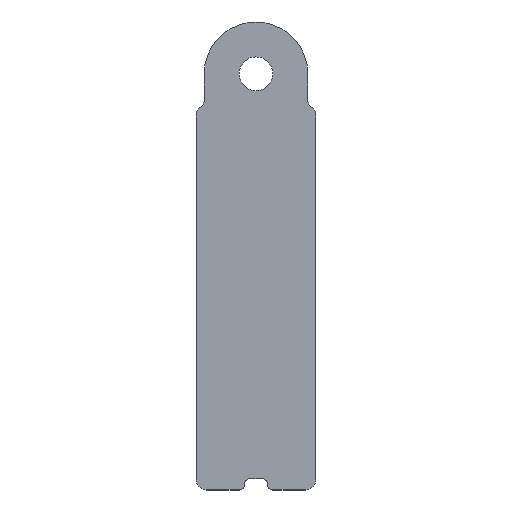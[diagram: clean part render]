
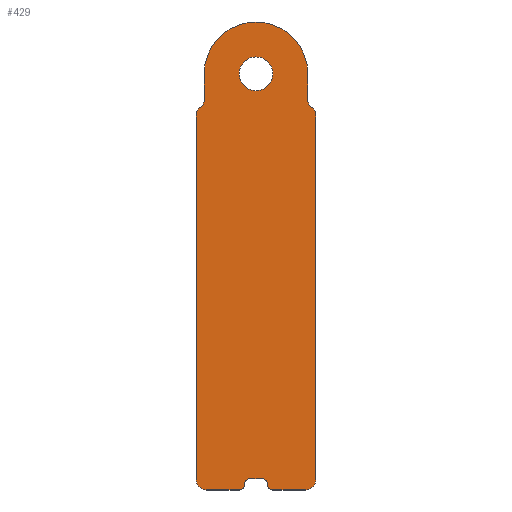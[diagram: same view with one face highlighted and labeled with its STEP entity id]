
A CAD part, top view. The second image highlights one B-rep face of the part: STEP entity #429.
In plain terms, the highlighted planar face has unit normal (0, 0, 1).
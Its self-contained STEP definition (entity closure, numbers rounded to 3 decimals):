
#16=FACE_BOUND('',#61,.T.);
#21=PLANE('',#482);
#36=FACE_OUTER_BOUND('',#60,.T.);
#60=EDGE_LOOP('',(#332,#333,#334,#335,#336,#337,#338,#339,#340,#341,#342,
#343,#344,#345,#346,#347,#348,#349,#350,#351));
#61=EDGE_LOOP('',(#352));
#87=LINE('',#692,#126);
#92=LINE('',#705,#131);
#95=LINE('',#714,#134);
#97=LINE('',#718,#136);
#98=LINE('',#722,#137);
#99=LINE('',#728,#138);
#100=LINE('',#732,#139);
#101=LINE('',#738,#140);
#102=LINE('',#740,#141);
#126=VECTOR('',#550,10.);
#131=VECTOR('',#565,10.);
#134=VECTOR('',#574,10.);
#136=VECTOR('',#578,10.);
#137=VECTOR('',#581,10.);
#138=VECTOR('',#586,10.);
#139=VECTOR('',#589,10.);
#140=VECTOR('',#594,10.);
#141=VECTOR('',#597,10.);
#154=CIRCLE('',#459,0.5);
#167=CIRCLE('',#475,0.5);
#168=CIRCLE('',#477,0.5);
#169=CIRCLE('',#480,0.5);
#170=CIRCLE('',#483,1.);
#171=CIRCLE('',#484,0.75);
#172=CIRCLE('',#485,0.75);
#173=CIRCLE('',#486,4.9);
#174=CIRCLE('',#487,0.75);
#175=CIRCLE('',#488,0.75);
#176=CIRCLE('',#489,1.);
#177=CIRCLE('',#490,1.6);
#178=VERTEX_POINT('',#642);
#179=VERTEX_POINT('',#643);
#201=VERTEX_POINT('',#691);
#202=VERTEX_POINT('',#695);
#203=VERTEX_POINT('',#699);
#204=VERTEX_POINT('',#701);
#205=VERTEX_POINT('',#707);
#206=VERTEX_POINT('',#708);
#207=VERTEX_POINT('',#713);
#208=VERTEX_POINT('',#717);
#209=VERTEX_POINT('',#719);
#210=VERTEX_POINT('',#721);
#211=VERTEX_POINT('',#723);
#212=VERTEX_POINT('',#725);
#213=VERTEX_POINT('',#727);
#214=VERTEX_POINT('',#729);
#215=VERTEX_POINT('',#731);
#216=VERTEX_POINT('',#733);
#217=VERTEX_POINT('',#735);
#218=VERTEX_POINT('',#737);
#219=VERTEX_POINT('',#741);
#220=EDGE_CURVE('',#178,#179,#154,.T.);
#244=EDGE_CURVE('',#201,#179,#87,.T.);
#246=EDGE_CURVE('',#201,#202,#167,.T.);
#249=EDGE_CURVE('',#203,#204,#168,.T.);
#251=EDGE_CURVE('',#203,#202,#92,.T.);
#252=EDGE_CURVE('',#205,#206,#169,.T.);
#255=EDGE_CURVE('',#207,#206,#95,.T.);
#257=EDGE_CURVE('',#178,#208,#97,.T.);
#258=EDGE_CURVE('',#209,#208,#170,.T.);
#259=EDGE_CURVE('',#209,#210,#98,.T.);
#260=EDGE_CURVE('',#211,#210,#171,.T.);
#261=EDGE_CURVE('',#212,#211,#172,.T.);
#262=EDGE_CURVE('',#212,#213,#99,.T.);
#263=EDGE_CURVE('',#213,#214,#173,.T.);
#264=EDGE_CURVE('',#214,#215,#100,.T.);
#265=EDGE_CURVE('',#216,#215,#174,.T.);
#266=EDGE_CURVE('',#217,#216,#175,.T.);
#267=EDGE_CURVE('',#217,#218,#101,.T.);
#268=EDGE_CURVE('',#207,#218,#176,.T.);
#269=EDGE_CURVE('',#205,#204,#102,.T.);
#270=EDGE_CURVE('',#219,#219,#177,.T.);
#332=ORIENTED_EDGE('',*,*,#220,.F.);
#333=ORIENTED_EDGE('',*,*,#257,.T.);
#334=ORIENTED_EDGE('',*,*,#258,.F.);
#335=ORIENTED_EDGE('',*,*,#259,.T.);
#336=ORIENTED_EDGE('',*,*,#260,.F.);
#337=ORIENTED_EDGE('',*,*,#261,.F.);
#338=ORIENTED_EDGE('',*,*,#262,.T.);
#339=ORIENTED_EDGE('',*,*,#263,.T.);
#340=ORIENTED_EDGE('',*,*,#264,.T.);
#341=ORIENTED_EDGE('',*,*,#265,.F.);
#342=ORIENTED_EDGE('',*,*,#266,.F.);
#343=ORIENTED_EDGE('',*,*,#267,.T.);
#344=ORIENTED_EDGE('',*,*,#268,.F.);
#345=ORIENTED_EDGE('',*,*,#255,.T.);
#346=ORIENTED_EDGE('',*,*,#252,.F.);
#347=ORIENTED_EDGE('',*,*,#269,.T.);
#348=ORIENTED_EDGE('',*,*,#249,.F.);
#349=ORIENTED_EDGE('',*,*,#251,.T.);
#350=ORIENTED_EDGE('',*,*,#246,.F.);
#351=ORIENTED_EDGE('',*,*,#244,.T.);
#352=ORIENTED_EDGE('',*,*,#270,.T.);
#429=ADVANCED_FACE('',(#36,#16),#21,.T.);
#459=AXIS2_PLACEMENT_3D('',#644,#509,#510);
#475=AXIS2_PLACEMENT_3D('',#696,#554,#555);
#477=AXIS2_PLACEMENT_3D('',#702,#560,#561);
#480=AXIS2_PLACEMENT_3D('',#709,#568,#569);
#482=AXIS2_PLACEMENT_3D('',#716,#576,#577);
#483=AXIS2_PLACEMENT_3D('',#720,#579,#580);
#484=AXIS2_PLACEMENT_3D('',#724,#582,#583);
#485=AXIS2_PLACEMENT_3D('',#726,#584,#585);
#486=AXIS2_PLACEMENT_3D('',#730,#587,#588);
#487=AXIS2_PLACEMENT_3D('',#734,#590,#591);
#488=AXIS2_PLACEMENT_3D('',#736,#592,#593);
#489=AXIS2_PLACEMENT_3D('',#739,#595,#596);
#490=AXIS2_PLACEMENT_3D('',#742,#598,#599);
#509=DIRECTION('center_axis',(0.,0.,-1.));
#510=DIRECTION('ref_axis',(-0.707,-0.707,0.));
#550=DIRECTION('',(0.,-1.,0.));
#554=DIRECTION('center_axis',(0.,0.,1.));
#555=DIRECTION('ref_axis',(0.707,0.707,0.));
#560=DIRECTION('center_axis',(0.,0.,1.));
#561=DIRECTION('ref_axis',(-0.707,0.707,0.));
#565=DIRECTION('',(1.,0.,0.));
#568=DIRECTION('center_axis',(0.,0.,-1.));
#569=DIRECTION('ref_axis',(0.707,-0.707,0.));
#574=DIRECTION('',(1.,0.,0.));
#576=DIRECTION('center_axis',(0.,0.,1.));
#577=DIRECTION('ref_axis',(1.,0.,0.));
#578=DIRECTION('',(1.,0.,0.));
#579=DIRECTION('center_axis',(0.,0.,-1.));
#580=DIRECTION('ref_axis',(0.707,-0.707,0.));
#581=DIRECTION('',(0.,1.,0.));
#582=DIRECTION('center_axis',(0.,0.,-1.));
#583=DIRECTION('ref_axis',(0.866,0.5,0.));
#584=DIRECTION('center_axis',(0.,0.,1.));
#585=DIRECTION('ref_axis',(-0.707,-0.707,0.));
#586=DIRECTION('',(0.,1.,0.));
#587=DIRECTION('center_axis',(0.,0.,1.));
#588=DIRECTION('ref_axis',(1.,0.,0.));
#589=DIRECTION('',(0.,-1.,0.));
#590=DIRECTION('center_axis',(0.,0.,1.));
#591=DIRECTION('ref_axis',(0.707,-0.707,0.));
#592=DIRECTION('center_axis',(0.,0.,-1.));
#593=DIRECTION('ref_axis',(-0.866,0.5,0.));
#594=DIRECTION('',(0.,-1.,0.));
#595=DIRECTION('center_axis',(0.,0.,-1.));
#596=DIRECTION('ref_axis',(-0.707,-0.707,0.));
#597=DIRECTION('',(0.,1.,0.));
#598=DIRECTION('center_axis',(0.,0.,-1.));
#599=DIRECTION('ref_axis',(1.,0.,0.));
#642=CARTESIAN_POINT('',(1.6,-39.35,1.8));
#643=CARTESIAN_POINT('',(1.1,-38.85,1.8));
#644=CARTESIAN_POINT('Origin',(1.6,-38.85,1.8));
#691=CARTESIAN_POINT('',(1.1,-38.8,1.8));
#692=CARTESIAN_POINT('',(1.1,-38.3,1.8));
#695=CARTESIAN_POINT('',(0.6,-38.3,1.8));
#696=CARTESIAN_POINT('Origin',(0.6,-38.8,1.8));
#699=CARTESIAN_POINT('',(-0.6,-38.3,1.8));
#701=CARTESIAN_POINT('',(-1.1,-38.8,1.8));
#702=CARTESIAN_POINT('Origin',(-0.6,-38.8,1.8));
#705=CARTESIAN_POINT('',(-1.1,-38.3,1.8));
#707=CARTESIAN_POINT('',(-1.1,-38.85,1.8));
#708=CARTESIAN_POINT('',(-1.6,-39.35,1.8));
#709=CARTESIAN_POINT('Origin',(-1.6,-38.85,1.8));
#713=CARTESIAN_POINT('',(-4.65,-39.35,1.8));
#714=CARTESIAN_POINT('',(-5.65,-39.35,1.8));
#716=CARTESIAN_POINT('Origin',(0.,-17.225,1.8));
#717=CARTESIAN_POINT('',(4.65,-39.35,1.8));
#718=CARTESIAN_POINT('',(-5.65,-39.35,1.8));
#719=CARTESIAN_POINT('',(5.65,-38.35,1.8));
#720=CARTESIAN_POINT('Origin',(4.65,-38.35,1.8));
#721=CARTESIAN_POINT('',(5.65,-3.799,1.8));
#722=CARTESIAN_POINT('',(5.65,-3.25,1.8));
#723=CARTESIAN_POINT('',(5.275,-3.15,1.8));
#724=CARTESIAN_POINT('Origin',(4.9,-3.799,1.8));
#725=CARTESIAN_POINT('',(4.9,-2.5,1.8));
#726=CARTESIAN_POINT('Origin',(5.65,-2.5,1.8));
#727=CARTESIAN_POINT('',(4.9,0.,1.8));
#728=CARTESIAN_POINT('',(4.9,0.,1.8));
#729=CARTESIAN_POINT('',(-4.9,0.,1.8));
#730=CARTESIAN_POINT('Origin',(0.,0.,1.8));
#731=CARTESIAN_POINT('',(-4.9,-2.5,1.8));
#732=CARTESIAN_POINT('',(-4.9,0.,1.8));
#733=CARTESIAN_POINT('',(-5.275,-3.15,1.8));
#734=CARTESIAN_POINT('Origin',(-5.65,-2.5,1.8));
#735=CARTESIAN_POINT('',(-5.65,-3.799,1.8));
#736=CARTESIAN_POINT('Origin',(-4.9,-3.799,1.8));
#737=CARTESIAN_POINT('',(-5.65,-38.35,1.8));
#738=CARTESIAN_POINT('',(-5.65,-3.25,1.8));
#739=CARTESIAN_POINT('Origin',(-4.65,-38.35,1.8));
#740=CARTESIAN_POINT('',(-1.1,-39.35,1.8));
#741=CARTESIAN_POINT('',(-1.6,0.,1.8));
#742=CARTESIAN_POINT('Origin',(0.,0.,1.8));
